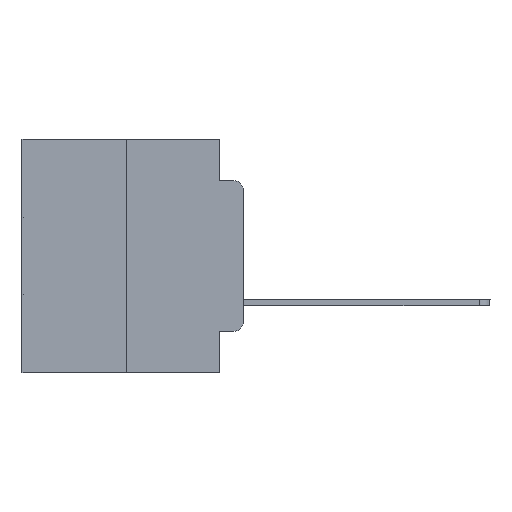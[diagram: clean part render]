
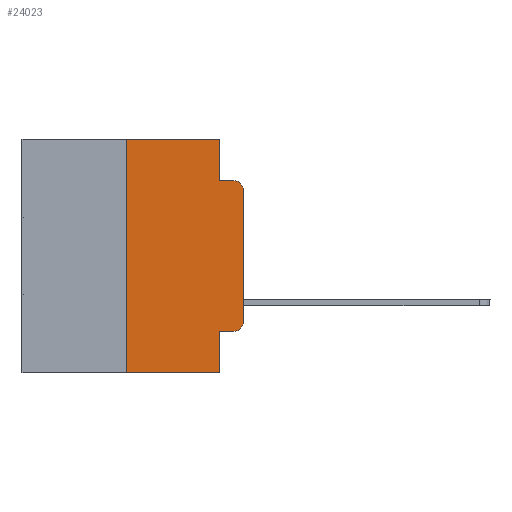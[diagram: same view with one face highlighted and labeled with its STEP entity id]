
A CAD part, left-side view. The second image highlights one B-rep face of the part: STEP entity #24023.
In plain terms, the highlighted planar face has unit normal (-1, 0, 0).
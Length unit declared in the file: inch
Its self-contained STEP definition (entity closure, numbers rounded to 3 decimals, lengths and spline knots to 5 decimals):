
#403 = LINE ( 'NONE', #2331, #9466 ) ;
#781 = CARTESIAN_POINT ( 'NONE',  ( 0., 0.051, -0.0885 ) ) ;
#959 = VERTEX_POINT ( 'NONE', #8777 ) ;
#1585 = CARTESIAN_POINT ( 'NONE',  ( 0., 0.051, -0.0885 ) ) ;
#2331 = CARTESIAN_POINT ( 'NONE',  ( 0., 0.473, 0. ) ) ;
#3087 = VERTEX_POINT ( 'NONE', #5233 ) ;
#3291 = CARTESIAN_POINT ( 'NONE',  ( 0., 0.473, -0.5 ) ) ;
#3393 = DIRECTION ( 'NONE',  ( 0., 0., 1. ) ) ;
#3548 = PLANE ( 'NONE',  #20651 ) ;
#3679 = CARTESIAN_POINT ( 'NONE',  ( 0., 0., 0. ) ) ;
#4003 = VERTEX_POINT ( 'NONE', #21065 ) ;
#4087 = VERTEX_POINT ( 'NONE', #19722 ) ;
#4484 = EDGE_CURVE ( 'NONE', #22167, #3087, #8507, .T. ) ;
#4827 = ORIENTED_EDGE ( 'NONE', *, *, #14639, .F. ) ;
#4949 = DIRECTION ( 'NONE',  ( 0., 0., -1. ) ) ;
#5113 = EDGE_CURVE ( 'NONE', #6338, #8739, #21558, .T. ) ;
#5191 = CARTESIAN_POINT ( 'NONE',  ( 0., 0., -0.3915 ) ) ;
#5233 = CARTESIAN_POINT ( 'NONE',  ( 0., 0.02, -0.0885 ) ) ;
#5474 = ORIENTED_EDGE ( 'NONE', *, *, #13371, .T. ) ;
#6131 = DIRECTION ( 'NONE',  ( 0., 0., -1. ) ) ;
#6338 = VERTEX_POINT ( 'NONE', #15380 ) ;
#7250 = ORIENTED_EDGE ( 'NONE', *, *, #12229, .T. ) ;
#7381 = DIRECTION ( 'NONE',  ( 0., 0., -1. ) ) ;
#8287 = EDGE_CURVE ( 'NONE', #6338, #4087, #11780, .T. ) ;
#8507 = LINE ( 'NONE', #1585, #28039 ) ;
#8519 = EDGE_LOOP ( 'NONE', ( #10859, #9875, #13132, #23308, #4827, #18603, #7250, #27143, #28895, #5474 ) ) ;
#8739 = VERTEX_POINT ( 'NONE', #28296 ) ;
#8777 = CARTESIAN_POINT ( 'NONE',  ( 0., 0., -0.1085 ) ) ;
#9234 = VECTOR ( 'NONE', #9590, 39.37008 ) ;
#9441 = EDGE_CURVE ( 'NONE', #20144, #11105, #14996, .T. ) ;
#9466 = VECTOR ( 'NONE', #15844, 39.37008 ) ;
#9482 = CARTESIAN_POINT ( 'NONE',  ( 0., 0.02, -0.3915 ) ) ;
#9580 = DIRECTION ( 'NONE',  ( -1., 0., 0. ) ) ;
#9590 = DIRECTION ( 'NONE',  ( 0., -1., 0. ) ) ;
#9875 = ORIENTED_EDGE ( 'NONE', *, *, #16535, .T. ) ;
#10307 = DIRECTION ( 'NONE',  ( 0., -1., 0. ) ) ;
#10395 = DIRECTION ( 'NONE',  ( 0., -1., 0. ) ) ;
#10859 = ORIENTED_EDGE ( 'NONE', *, *, #28547, .T. ) ;
#10928 = DIRECTION ( 'NONE',  ( 0., 0., -1. ) ) ;
#11105 = VERTEX_POINT ( 'NONE', #26436 ) ;
#11780 = LINE ( 'NONE', #27379, #9234 ) ;
#12087 = VECTOR ( 'NONE', #12938, 39.37008 ) ;
#12229 = EDGE_CURVE ( 'NONE', #20144, #8739, #21655, .T. ) ;
#12270 = VECTOR ( 'NONE', #10928, 39.37008 ) ;
#12938 = DIRECTION ( 'NONE',  ( 0., 0., 1. ) ) ;
#13132 = ORIENTED_EDGE ( 'NONE', *, *, #4484, .F. ) ;
#13136 = CIRCLE ( 'NONE', #26777, 0.02 ) ;
#13371 = EDGE_CURVE ( 'NONE', #4087, #22552, #13136, .T. ) ;
#13838 = CARTESIAN_POINT ( 'NONE',  ( 0., 0.02, -0.1085 ) ) ;
#14639 = EDGE_CURVE ( 'NONE', #11105, #4003, #403, .T. ) ;
#14701 = FACE_OUTER_BOUND ( 'NONE', #8519, .T. ) ;
#14996 = LINE ( 'NONE', #15155, #12087 ) ;
#15155 = CARTESIAN_POINT ( 'NONE',  ( 0., 0.25, 0. ) ) ;
#15380 = CARTESIAN_POINT ( 'NONE',  ( 0., 0.051, -0.4115 ) ) ;
#15790 = CARTESIAN_POINT ( 'NONE',  ( 0., 0.051, 0. ) ) ;
#15844 = DIRECTION ( 'NONE',  ( 0., -1., 0. ) ) ;
#16247 = DIRECTION ( 'NONE',  ( -1., 0., 0. ) ) ;
#16535 = EDGE_CURVE ( 'NONE', #959, #3087, #24990, .T. ) ;
#17997 = LINE ( 'NONE', #15790, #12270 ) ;
#18603 = ORIENTED_EDGE ( 'NONE', *, *, #9441, .F. ) ;
#19354 = CARTESIAN_POINT ( 'NONE',  ( 0., 0.051, 0. ) ) ;
#19722 = CARTESIAN_POINT ( 'NONE',  ( 0., 0.02, -0.4115 ) ) ;
#20144 = VERTEX_POINT ( 'NONE', #24074 ) ;
#20651 = AXIS2_PLACEMENT_3D ( 'NONE', #28072, #21474, #27278 ) ;
#21065 = CARTESIAN_POINT ( 'NONE',  ( 0., 0.051, 0. ) ) ;
#21474 = DIRECTION ( 'NONE',  ( 1., 0., 0. ) ) ;
#21558 = LINE ( 'NONE', #19354, #23293 ) ;
#21655 = LINE ( 'NONE', #3291, #24852 ) ;
#22167 = VERTEX_POINT ( 'NONE', #781 ) ;
#22552 = VERTEX_POINT ( 'NONE', #5191 ) ;
#22660 = VECTOR ( 'NONE', #3393, 39.37008 ) ;
#23143 = AXIS2_PLACEMENT_3D ( 'NONE', #13838, #9580, #7381 ) ;
#23293 = VECTOR ( 'NONE', #6131, 39.37008 ) ;
#23308 = ORIENTED_EDGE ( 'NONE', *, *, #27821, .F. ) ;
#24023 = ADVANCED_FACE ( 'NONE', ( #14701 ), #3548, .F. ) ;
#24074 = CARTESIAN_POINT ( 'NONE',  ( 0., 0.25, -0.5 ) ) ;
#24852 = VECTOR ( 'NONE', #10307, 39.37008 ) ;
#24990 = CIRCLE ( 'NONE', #23143, 0.02 ) ;
#25852 = LINE ( 'NONE', #3679, #22660 ) ;
#26436 = CARTESIAN_POINT ( 'NONE',  ( 0., 0.25, 0. ) ) ;
#26777 = AXIS2_PLACEMENT_3D ( 'NONE', #9482, #16247, #4949 ) ;
#27143 = ORIENTED_EDGE ( 'NONE', *, *, #5113, .F. ) ;
#27278 = DIRECTION ( 'NONE',  ( 0., 0., -1. ) ) ;
#27379 = CARTESIAN_POINT ( 'NONE',  ( 0., 0.051, -0.4115 ) ) ;
#27821 = EDGE_CURVE ( 'NONE', #4003, #22167, #17997, .T. ) ;
#28039 = VECTOR ( 'NONE', #10395, 39.37008 ) ;
#28072 = CARTESIAN_POINT ( 'NONE',  ( 0., 0.473, 0. ) ) ;
#28296 = CARTESIAN_POINT ( 'NONE',  ( 0., 0.051, -0.5 ) ) ;
#28547 = EDGE_CURVE ( 'NONE', #22552, #959, #25852, .T. ) ;
#28895 = ORIENTED_EDGE ( 'NONE', *, *, #8287, .T. ) ;
